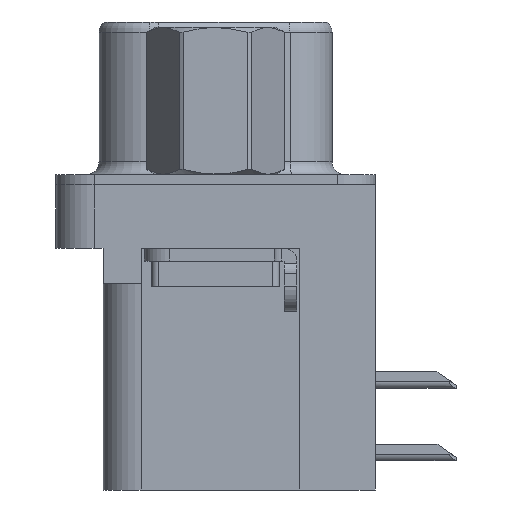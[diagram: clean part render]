
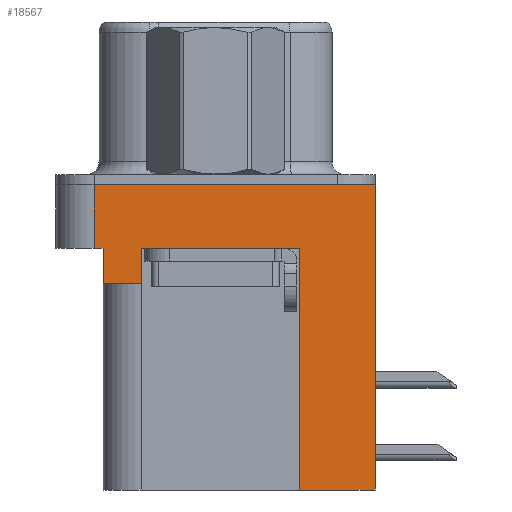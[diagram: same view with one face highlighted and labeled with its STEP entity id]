
A CAD part, left-side view. The second image highlights one B-rep face of the part: STEP entity #18567.
In plain terms, the highlighted planar face has unit normal (-1, 0, 0).
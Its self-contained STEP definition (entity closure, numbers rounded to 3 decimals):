
#353 = CARTESIAN_POINT ( 'NONE',  ( -2.935, 4.775, -2.5 ) ) ;
#609 = DIRECTION ( 'NONE',  ( 0., 0., 1. ) ) ;
#633 = ORIENTED_EDGE ( 'NONE', *, *, #23289, .F. ) ;
#893 = ORIENTED_EDGE ( 'NONE', *, *, #14486, .F. ) ;
#1001 = VERTEX_POINT ( 'NONE', #13299 ) ;
#1429 = VERTEX_POINT ( 'NONE', #14772 ) ;
#1470 = EDGE_CURVE ( 'NONE', #19332, #5265, #5902, .T. ) ;
#3592 = CARTESIAN_POINT ( 'NONE',  ( -2.935, -6.275, -2.5 ) ) ;
#3623 = ORIENTED_EDGE ( 'NONE', *, *, #18115, .T. ) ;
#4039 = VECTOR ( 'NONE', #7031, 1000. ) ;
#4092 = LINE ( 'NONE', #5101, #4039 ) ;
#4337 = VECTOR ( 'NONE', #4468, 1000. ) ;
#4468 = DIRECTION ( 'NONE',  ( 0., 0., 1. ) ) ;
#4529 = ORIENTED_EDGE ( 'NONE', *, *, #13775, .T. ) ;
#4702 = LINE ( 'NONE', #353, #4337 ) ;
#5101 = CARTESIAN_POINT ( 'NONE',  ( -2.935, 4.425, -3.9 ) ) ;
#5209 = CARTESIAN_POINT ( 'NONE',  ( -2.935, -6.275, -2.5 ) ) ;
#5233 = DIRECTION ( 'NONE',  ( 0., 0., 1. ) ) ;
#5265 = VERTEX_POINT ( 'NONE', #21389 ) ;
#5339 = VERTEX_POINT ( 'NONE', #15313 ) ;
#5749 = VECTOR ( 'NONE', #10269, 1000. ) ;
#5843 = ORIENTED_EDGE ( 'NONE', *, *, #1470, .F. ) ;
#5902 = LINE ( 'NONE', #11906, #5749 ) ;
#6076 = VECTOR ( 'NONE', #11733, 1000. ) ;
#6142 = LINE ( 'NONE', #13587, #6076 ) ;
#6324 = VERTEX_POINT ( 'NONE', #13096 ) ;
#6903 = VECTOR ( 'NONE', #9078, 1000. ) ;
#6906 = CARTESIAN_POINT ( 'NONE',  ( -2.935, -6.275, -2.5 ) ) ;
#7031 = DIRECTION ( 'NONE',  ( 0., 1., 0. ) ) ;
#7324 = LINE ( 'NONE', #5209, #6903 ) ;
#8139 = DIRECTION ( 'NONE',  ( 0., -1., 0. ) ) ;
#8626 = ORIENTED_EDGE ( 'NONE', *, *, #13179, .F. ) ;
#8812 = CARTESIAN_POINT ( 'NONE',  ( -2.935, -6.275, -2.5 ) ) ;
#9078 = DIRECTION ( 'NONE',  ( 0., 0., 1. ) ) ;
#9791 = FACE_OUTER_BOUND ( 'NONE', #21939, .T. ) ;
#9857 = VERTEX_POINT ( 'NONE', #14436 ) ;
#10206 = VECTOR ( 'NONE', #5233, 1000. ) ;
#10250 = LINE ( 'NONE', #17984, #10206 ) ;
#10269 = DIRECTION ( 'NONE',  ( 0., 0., 1. ) ) ;
#10729 = PLANE ( 'NONE',  #14942 ) ;
#11032 = ORIENTED_EDGE ( 'NONE', *, *, #19264, .F. ) ;
#11733 = DIRECTION ( 'NONE',  ( 0., 1., 0. ) ) ;
#11857 = VECTOR ( 'NONE', #16528, 1000. ) ;
#11879 = LINE ( 'NONE', #3592, #11857 ) ;
#11906 = CARTESIAN_POINT ( 'NONE',  ( -2.935, 4.425, -3.9 ) ) ;
#12295 = VERTEX_POINT ( 'NONE', #12550 ) ;
#12550 = CARTESIAN_POINT ( 'NONE',  ( -2.935, -3.295, -2.5 ) ) ;
#12572 = DIRECTION ( 'NONE',  ( 0., 0., 1. ) ) ;
#12659 = VERTEX_POINT ( 'NONE', #16621 ) ;
#12782 = ORIENTED_EDGE ( 'NONE', *, *, #17899, .T. ) ;
#12816 = VECTOR ( 'NONE', #609, 1000. ) ;
#12868 = LINE ( 'NONE', #19200, #12816 ) ;
#13096 = CARTESIAN_POINT ( 'NONE',  ( -2.935, -6.275, 0. ) ) ;
#13179 = EDGE_CURVE ( 'NONE', #12659, #12295, #10250, .T. ) ;
#13191 = VERTEX_POINT ( 'NONE', #14620 ) ;
#13299 = CARTESIAN_POINT ( 'NONE',  ( -2.935, -6.275, -12. ) ) ;
#13572 = LINE ( 'NONE', #8812, #13718 ) ;
#13587 = CARTESIAN_POINT ( 'NONE',  ( -2.935, -3.295, -12. ) ) ;
#13718 = VECTOR ( 'NONE', #21277, 1000. ) ;
#13775 = EDGE_CURVE ( 'NONE', #1001, #6324, #7324, .T. ) ;
#14436 = CARTESIAN_POINT ( 'NONE',  ( -2.935, 4.775, 0. ) ) ;
#14486 = EDGE_CURVE ( 'NONE', #5339, #19332, #4092, .T. ) ;
#14620 = CARTESIAN_POINT ( 'NONE',  ( -2.935, 4.775, -2.5 ) ) ;
#14772 = CARTESIAN_POINT ( 'NONE',  ( -2.935, 2.895, -2.5 ) ) ;
#14942 = AXIS2_PLACEMENT_3D ( 'NONE', #6906, #22917, #12572 ) ;
#15313 = CARTESIAN_POINT ( 'NONE',  ( -2.935, 2.895, -3.9 ) ) ;
#16528 = DIRECTION ( 'NONE',  ( 0., -1., 0. ) ) ;
#16621 = CARTESIAN_POINT ( 'NONE',  ( -2.935, -3.295, -12. ) ) ;
#17899 = EDGE_CURVE ( 'NONE', #5339, #1429, #12868, .T. ) ;
#17984 = CARTESIAN_POINT ( 'NONE',  ( -2.935, -3.295, -12. ) ) ;
#18115 = EDGE_CURVE ( 'NONE', #13191, #5265, #11879, .T. ) ;
#18567 = ADVANCED_FACE ( 'NONE', ( #9791 ), #10729, .T. ) ;
#18859 = CARTESIAN_POINT ( 'NONE',  ( -2.935, -6.275, 0. ) ) ;
#19139 = CARTESIAN_POINT ( 'NONE',  ( -2.935, 4.425, -3.9 ) ) ;
#19200 = CARTESIAN_POINT ( 'NONE',  ( -2.935, 2.895, -3.9 ) ) ;
#19264 = EDGE_CURVE ( 'NONE', #13191, #9857, #4702, .T. ) ;
#19332 = VERTEX_POINT ( 'NONE', #19139 ) ;
#19873 = VECTOR ( 'NONE', #8139, 1000. ) ;
#19893 = LINE ( 'NONE', #18859, #19873 ) ;
#20779 = ORIENTED_EDGE ( 'NONE', *, *, #23617, .T. ) ;
#20828 = ORIENTED_EDGE ( 'NONE', *, *, #22011, .F. ) ;
#21277 = DIRECTION ( 'NONE',  ( 0., -1., 0. ) ) ;
#21389 = CARTESIAN_POINT ( 'NONE',  ( -2.935, 4.425, -2.5 ) ) ;
#21939 = EDGE_LOOP ( 'NONE', ( #633, #11032, #3623, #5843, #893, #12782, #20779, #8626, #20828, #4529 ) ) ;
#22011 = EDGE_CURVE ( 'NONE', #1001, #12659, #6142, .T. ) ;
#22917 = DIRECTION ( 'NONE',  ( -1., 0., 0. ) ) ;
#23289 = EDGE_CURVE ( 'NONE', #9857, #6324, #19893, .T. ) ;
#23617 = EDGE_CURVE ( 'NONE', #1429, #12295, #13572, .T. ) ;
